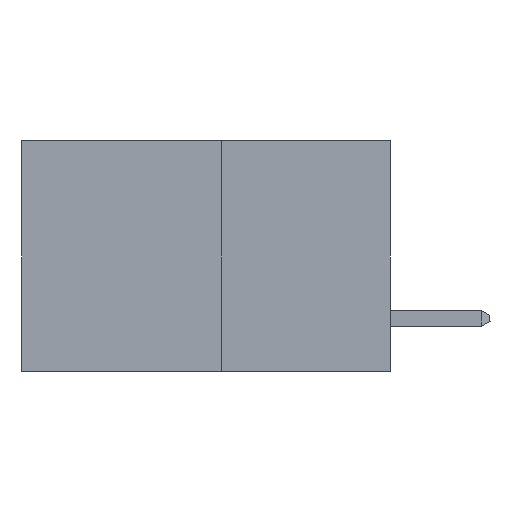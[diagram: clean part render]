
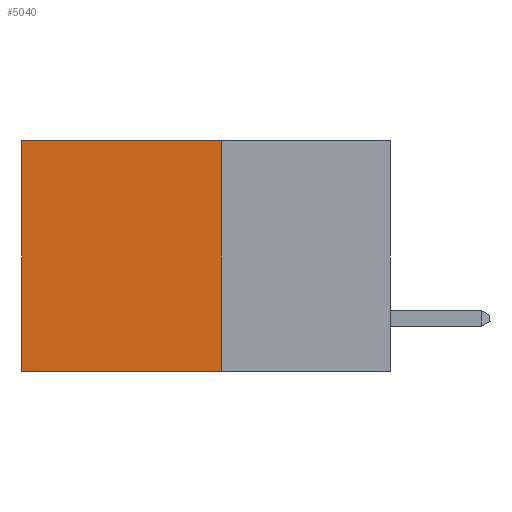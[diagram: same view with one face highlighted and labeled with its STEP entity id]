
A CAD part, left-side view. The second image highlights one B-rep face of the part: STEP entity #5040.
In plain terms, the highlighted planar face has unit normal (-1, 0, 0).
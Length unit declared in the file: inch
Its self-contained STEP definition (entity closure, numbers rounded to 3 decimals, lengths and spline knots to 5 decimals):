
#202 = DIRECTION ( 'NONE',  ( 0., 0., -1. ) ) ;
#281 = FACE_OUTER_BOUND ( 'NONE', #13568, .T. ) ;
#405 = EDGE_CURVE ( 'NONE', #8989, #7689, #9278, .T. ) ;
#1023 = CARTESIAN_POINT ( 'NONE',  ( 0.277, 0.27, -0.37 ) ) ;
#1329 = EDGE_CURVE ( 'NONE', #14755, #7689, #2268, .T. ) ;
#2049 = AXIS2_PLACEMENT_3D ( 'NONE', #14434, #13244, #9421 ) ;
#2232 = ORIENTED_EDGE ( 'NONE', *, *, #4146, .F. ) ;
#2268 = LINE ( 'NONE', #14098, #11599 ) ;
#2275 = VECTOR ( 'NONE', #10689, 39.37008 ) ;
#2623 = ORIENTED_EDGE ( 'NONE', *, *, #5104, .T. ) ;
#3055 = LINE ( 'NONE', #6511, #5832 ) ;
#3220 = CARTESIAN_POINT ( 'NONE',  ( 0.277, 0.27, 0. ) ) ;
#3489 = DIRECTION ( 'NONE',  ( 0., 0., -1. ) ) ;
#3653 = ORIENTED_EDGE ( 'NONE', *, *, #1329, .T. ) ;
#4146 = EDGE_CURVE ( 'NONE', #9503, #8989, #3055, .T. ) ;
#5040 = ADVANCED_FACE ( 'NONE', ( #281 ), #14287, .F. ) ;
#5104 = EDGE_CURVE ( 'NONE', #9503, #14755, #8566, .T. ) ;
#5832 = VECTOR ( 'NONE', #3489, 39.37008 ) ;
#6511 = CARTESIAN_POINT ( 'NONE',  ( 0.277, 0.27, -0.37 ) ) ;
#7689 = VERTEX_POINT ( 'NONE', #11681 ) ;
#8275 = CARTESIAN_POINT ( 'NONE',  ( 0.277, 0.27, 0. ) ) ;
#8566 = LINE ( 'NONE', #3220, #2275 ) ;
#8989 = VERTEX_POINT ( 'NONE', #13051 ) ;
#9278 = LINE ( 'NONE', #1023, #12331 ) ;
#9421 = DIRECTION ( 'NONE',  ( 0., 0., -1. ) ) ;
#9503 = VERTEX_POINT ( 'NONE', #8275 ) ;
#10689 = DIRECTION ( 'NONE',  ( 0., 1., 0. ) ) ;
#10691 = CARTESIAN_POINT ( 'NONE',  ( 0.277, 0.59, 0. ) ) ;
#11153 = DIRECTION ( 'NONE',  ( 0., 1., 0. ) ) ;
#11599 = VECTOR ( 'NONE', #202, 39.37008 ) ;
#11681 = CARTESIAN_POINT ( 'NONE',  ( 0.277, 0.59, -0.37 ) ) ;
#12331 = VECTOR ( 'NONE', #11153, 39.37008 ) ;
#13051 = CARTESIAN_POINT ( 'NONE',  ( 0.277, 0.27, -0.37 ) ) ;
#13244 = DIRECTION ( 'NONE',  ( 1., 0., 0. ) ) ;
#13568 = EDGE_LOOP ( 'NONE', ( #3653, #14539, #2232, #2623 ) ) ;
#14098 = CARTESIAN_POINT ( 'NONE',  ( 0.277, 0.59, -0.37 ) ) ;
#14287 = PLANE ( 'NONE',  #2049 ) ;
#14434 = CARTESIAN_POINT ( 'NONE',  ( 0.277, 0.27, -0.37 ) ) ;
#14539 = ORIENTED_EDGE ( 'NONE', *, *, #405, .F. ) ;
#14755 = VERTEX_POINT ( 'NONE', #10691 ) ;
